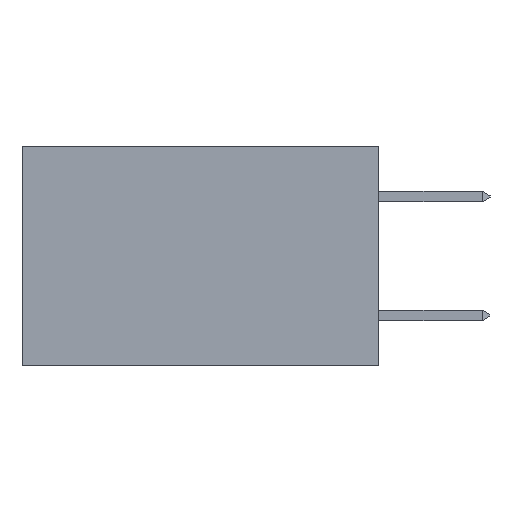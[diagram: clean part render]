
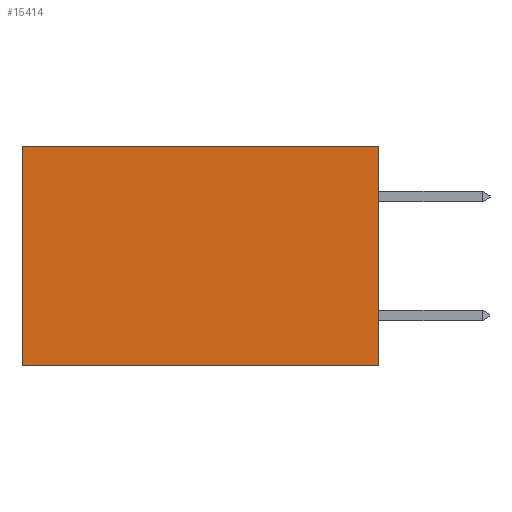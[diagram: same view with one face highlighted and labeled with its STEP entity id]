
A CAD part, left-side view. The second image highlights one B-rep face of the part: STEP entity #15414.
In plain terms, the highlighted planar face has unit normal (-1, 0, 0).
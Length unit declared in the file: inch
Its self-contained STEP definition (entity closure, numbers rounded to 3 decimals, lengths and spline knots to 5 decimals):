
#38 = VERTEX_POINT ( 'NONE', #20218 ) ;
#789 = VERTEX_POINT ( 'NONE', #803 ) ;
#803 = CARTESIAN_POINT ( 'NONE',  ( 0.298, 0., -0.37 ) ) ;
#980 = DIRECTION ( 'NONE',  ( 0., 0., -1. ) ) ;
#1692 = FACE_OUTER_BOUND ( 'NONE', #7761, .T. ) ;
#2190 = ORIENTED_EDGE ( 'NONE', *, *, #9611, .F. ) ;
#2657 = EDGE_CURVE ( 'NONE', #38, #5766, #14709, .T. ) ;
#3162 = CARTESIAN_POINT ( 'NONE',  ( 0.298, 0., 0. ) ) ;
#3580 = CARTESIAN_POINT ( 'NONE',  ( 0.298, 0.6, -0.37 ) ) ;
#5500 = LINE ( 'NONE', #23304, #10393 ) ;
#5766 = VERTEX_POINT ( 'NONE', #3580 ) ;
#6454 = ORIENTED_EDGE ( 'NONE', *, *, #11100, .F. ) ;
#6927 = CARTESIAN_POINT ( 'NONE',  ( 0.298, 0., 0. ) ) ;
#7761 = EDGE_LOOP ( 'NONE', ( #18570, #2190, #6454, #18196 ) ) ;
#8783 = DIRECTION ( 'NONE',  ( 0., 0., -1. ) ) ;
#9365 = VECTOR ( 'NONE', #9783, 39.37008 ) ;
#9611 = EDGE_CURVE ( 'NONE', #789, #5766, #13536, .T. ) ;
#9783 = DIRECTION ( 'NONE',  ( 0., 0., -1. ) ) ;
#10393 = VECTOR ( 'NONE', #10891, 39.37008 ) ;
#10553 = LINE ( 'NONE', #18772, #9365 ) ;
#10891 = DIRECTION ( 'NONE',  ( 0., 1., 0. ) ) ;
#11100 = EDGE_CURVE ( 'NONE', #15366, #789, #10553, .T. ) ;
#12954 = VECTOR ( 'NONE', #21491, 39.37008 ) ;
#13536 = LINE ( 'NONE', #14412, #12954 ) ;
#13602 = CARTESIAN_POINT ( 'NONE',  ( 0.298, 0.6, 0. ) ) ;
#14104 = EDGE_CURVE ( 'NONE', #15366, #38, #5500, .T. ) ;
#14298 = PLANE ( 'NONE',  #20925 ) ;
#14412 = CARTESIAN_POINT ( 'NONE',  ( 0.298, 0., -0.37 ) ) ;
#14709 = LINE ( 'NONE', #13602, #18823 ) ;
#15366 = VERTEX_POINT ( 'NONE', #3162 ) ;
#15414 = ADVANCED_FACE ( 'NONE', ( #1692 ), #14298, .F. ) ;
#18196 = ORIENTED_EDGE ( 'NONE', *, *, #14104, .T. ) ;
#18570 = ORIENTED_EDGE ( 'NONE', *, *, #2657, .T. ) ;
#18772 = CARTESIAN_POINT ( 'NONE',  ( 0.298, 0., 0. ) ) ;
#18823 = VECTOR ( 'NONE', #980, 39.37008 ) ;
#19593 = DIRECTION ( 'NONE',  ( 1., 0., 0. ) ) ;
#20218 = CARTESIAN_POINT ( 'NONE',  ( 0.298, 0.6, 0. ) ) ;
#20925 = AXIS2_PLACEMENT_3D ( 'NONE', #6927, #19593, #8783 ) ;
#21491 = DIRECTION ( 'NONE',  ( 0., 1., 0. ) ) ;
#23304 = CARTESIAN_POINT ( 'NONE',  ( 0.298, 0., 0. ) ) ;
